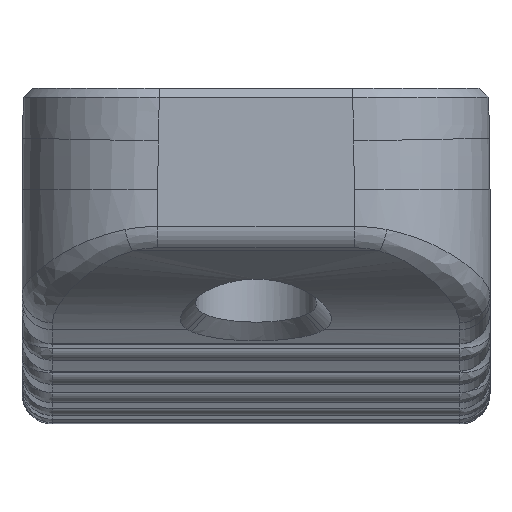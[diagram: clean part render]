
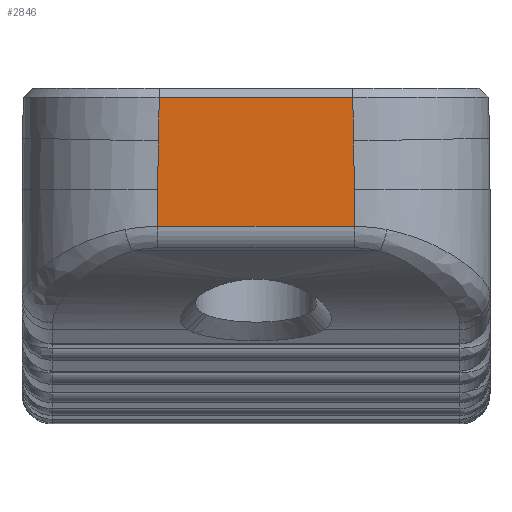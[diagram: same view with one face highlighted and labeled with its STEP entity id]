
A CAD part, top view. The second image highlights one B-rep face of the part: STEP entity #2846.
In plain terms, the highlighted planar face has unit normal (0, 0, 1).
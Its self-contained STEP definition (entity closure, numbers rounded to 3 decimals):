
#92=CIRCLE('',#2902,3191.507);
#262=CIRCLE('',#3183,156.5);
#263=CIRCLE('',#3184,156.5);
#264=CIRCLE('',#3185,3191.507);
#344=B_SPLINE_CURVE_WITH_KNOTS('',3,(#4262,#4263,#4264,#4265),
 .UNSPECIFIED.,.F.,.F.,(4,4),(-3.999,-3.998),
 .UNSPECIFIED.);
#350=B_SPLINE_CURVE_WITH_KNOTS('',3,(#4547,#4548,#4549,#4550),
 .UNSPECIFIED.,.F.,.F.,(4,4),(-1.334,-1.333),
 .UNSPECIFIED.);
#705=FACE_OUTER_BOUND('',#909,.T.);
#909=EDGE_LOOP('',(#2455,#2456,#2457,#2458,#2459,#2460,#2461,#2462,#2463,
#2464));
#953=LINE('',#4242,#1053);
#971=LINE('',#8833,#1071);
#1019=LINE('',#9119,#1119);
#1021=LINE('',#9126,#1121);
#1053=VECTOR('',#3242,10.);
#1071=VECTOR('',#3594,10.);
#1119=VECTOR('',#3876,10.);
#1121=VECTOR('',#3884,10.);
#1151=VERTEX_POINT('',#4070);
#1155=VERTEX_POINT('',#4239);
#1156=VERTEX_POINT('',#4241);
#1158=VERTEX_POINT('',#4374);
#1171=VERTEX_POINT('',#4615);
#1334=VERTEX_POINT('',#8825);
#1336=VERTEX_POINT('',#8831);
#1347=VERTEX_POINT('',#9118);
#1349=VERTEX_POINT('',#9125);
#1350=VERTEX_POINT('',#9127);
#1387=EDGE_CURVE('',#1155,#1156,#953,.T.);
#1390=EDGE_CURVE('',#1156,#1151,#344,.T.);
#1402=EDGE_CURVE('',#1158,#1155,#350,.T.);
#1414=EDGE_CURVE('',#1171,#1158,#92,.T.);
#1641=EDGE_CURVE('',#1336,#1334,#971,.T.);
#1744=EDGE_CURVE('',#1334,#1347,#1019,.T.);
#1747=EDGE_CURVE('',#1347,#1171,#262,.T.);
#1748=EDGE_CURVE('',#1349,#1336,#1021,.T.);
#1749=EDGE_CURVE('',#1350,#1349,#263,.T.);
#1750=EDGE_CURVE('',#1151,#1350,#264,.T.);
#2455=ORIENTED_EDGE('',*,*,#1402,.F.);
#2456=ORIENTED_EDGE('',*,*,#1414,.F.);
#2457=ORIENTED_EDGE('',*,*,#1747,.F.);
#2458=ORIENTED_EDGE('',*,*,#1744,.F.);
#2459=ORIENTED_EDGE('',*,*,#1641,.F.);
#2460=ORIENTED_EDGE('',*,*,#1748,.F.);
#2461=ORIENTED_EDGE('',*,*,#1749,.F.);
#2462=ORIENTED_EDGE('',*,*,#1750,.F.);
#2463=ORIENTED_EDGE('',*,*,#1390,.F.);
#2464=ORIENTED_EDGE('',*,*,#1387,.F.);
#2673=PLANE('',#3182);
#2846=ADVANCED_FACE('',(#705),#2673,.T.);
#2902=AXIS2_PLACEMENT_3D('',#4617,#3265,#3266);
#3182=AXIS2_PLACEMENT_3D('',#9123,#3880,#3881);
#3183=AXIS2_PLACEMENT_3D('',#9124,#3882,#3883);
#3184=AXIS2_PLACEMENT_3D('',#9128,#3885,#3886);
#3185=AXIS2_PLACEMENT_3D('',#9129,#3887,#3888);
#3242=DIRECTION('',(1.,0.,0.));
#3265=DIRECTION('center_axis',(0.,0.,1.));
#3266=DIRECTION('ref_axis',(1.,-0.004,0.));
#3594=DIRECTION('',(-1.,0.,0.));
#3876=DIRECTION('',(0.,1.,0.));
#3880=DIRECTION('center_axis',(0.,0.,1.));
#3881=DIRECTION('ref_axis',(0.,1.,0.));
#3882=DIRECTION('center_axis',(0.,0.,-1.));
#3883=DIRECTION('ref_axis',(-1.,0.01,0.));
#3884=DIRECTION('',(0.,-1.,0.));
#3885=DIRECTION('center_axis',(0.,0.,-1.));
#3886=DIRECTION('ref_axis',(1.,0.01,0.));
#3887=DIRECTION('center_axis',(0.,0.,1.));
#3888=DIRECTION('ref_axis',(-1.,-0.004,0.));
#4070=CARTESIAN_POINT('',(22.385,399.4,-120.588));
#4239=CARTESIAN_POINT('',(9.58,399.4,-120.588));
#4241=CARTESIAN_POINT('',(22.374,399.4,-120.588));
#4242=CARTESIAN_POINT('',(24.727,399.4,-120.588));
#4262=CARTESIAN_POINT('Ctrl Pts',(22.374,399.4,-120.588));
#4263=CARTESIAN_POINT('Ctrl Pts',(22.378,399.4,-120.588));
#4264=CARTESIAN_POINT('Ctrl Pts',(22.381,399.4,-120.588));
#4265=CARTESIAN_POINT('Ctrl Pts',(22.385,399.4,-120.588));
#4374=CARTESIAN_POINT('',(9.568,399.4,-120.588));
#4547=CARTESIAN_POINT('Ctrl Pts',(9.568,399.4,-120.588));
#4548=CARTESIAN_POINT('Ctrl Pts',(9.572,399.4,-120.588));
#4549=CARTESIAN_POINT('Ctrl Pts',(9.576,399.4,-120.588));
#4550=CARTESIAN_POINT('Ctrl Pts',(9.58,399.4,-120.588));
#4615=CARTESIAN_POINT('',(9.51,396.491,-120.588));
#4617=CARTESIAN_POINT('Origin',(-3181.326,461.945,-120.588));
#8825=CARTESIAN_POINT('',(9.477,390.828,-120.588));
#8831=CARTESIAN_POINT('',(22.477,390.828,-120.588));
#8833=CARTESIAN_POINT('',(33.477,390.828,-120.588));
#9118=CARTESIAN_POINT('',(9.477,393.281,-120.588));
#9119=CARTESIAN_POINT('',(9.477,420.5,-120.588));
#9123=CARTESIAN_POINT('Origin',(33.477,446.,-120.588));
#9124=CARTESIAN_POINT('Origin',(165.977,393.281,-120.588));
#9125=CARTESIAN_POINT('',(22.477,393.281,-120.588));
#9126=CARTESIAN_POINT('',(22.477,413.,-120.588));
#9127=CARTESIAN_POINT('',(22.444,396.491,-120.588));
#9128=CARTESIAN_POINT('Origin',(-134.023,393.281,-120.588));
#9129=CARTESIAN_POINT('Origin',(3213.279,461.945,-120.588));
